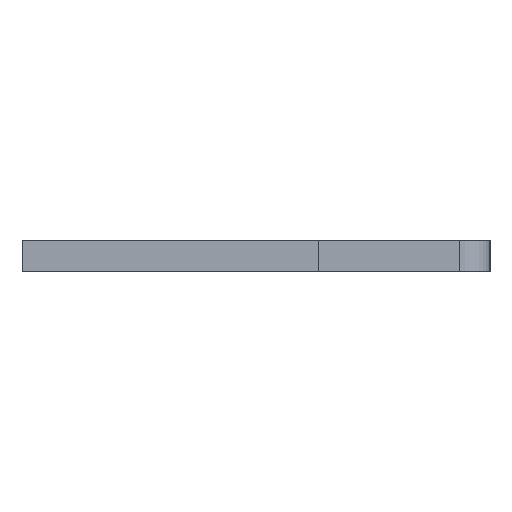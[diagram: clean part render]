
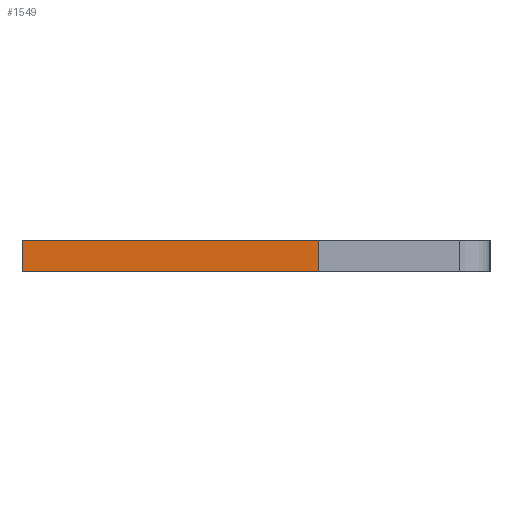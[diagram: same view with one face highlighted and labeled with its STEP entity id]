
A CAD part, left-side view. The second image highlights one B-rep face of the part: STEP entity #1549.
In plain terms, the highlighted face is planar.
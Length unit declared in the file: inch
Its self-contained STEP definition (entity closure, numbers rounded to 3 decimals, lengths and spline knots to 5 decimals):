
#20 = CARTESIAN_POINT ( 'NONE',  ( -0.01, 0.15, -0.04 ) ) ;
#60 = CARTESIAN_POINT ( 'NONE',  ( 0.01, 0.15, -0.04 ) ) ;
#289 = LINE ( 'NONE', #20, #526 ) ;
#394 = LINE ( 'NONE', #60, #2786 ) ;
#432 = CARTESIAN_POINT ( 'NONE',  ( 0.01, -0.04, -0.04 ) ) ;
#434 = VERTEX_POINT ( 'NONE', #1658 ) ;
#450 = DIRECTION ( 'NONE',  ( 1., 0., 0. ) ) ;
#476 = DIRECTION ( 'NONE',  ( 0., 1., 0. ) ) ;
#503 = ORIENTED_EDGE ( 'NONE', *, *, #1906, .T. ) ;
#526 = VECTOR ( 'NONE', #476, 39.37008 ) ;
#716 = ORIENTED_EDGE ( 'NONE', *, *, #2510, .F. ) ;
#841 = VERTEX_POINT ( 'NONE', #861 ) ;
#842 = VECTOR ( 'NONE', #1188, 39.37008 ) ;
#861 = CARTESIAN_POINT ( 'NONE',  ( 0.01, -0.04, -0.04 ) ) ;
#869 = DIRECTION ( 'NONE',  ( -1., 0., 0. ) ) ;
#949 = LINE ( 'NONE', #432, #1327 ) ;
#1083 = PLANE ( 'NONE',  #2396 ) ;
#1135 = CARTESIAN_POINT ( 'NONE',  ( 0.01, 0.15, -0.04 ) ) ;
#1148 = LINE ( 'NONE', #1591, #842 ) ;
#1166 = DIRECTION ( 'NONE',  ( -1., 0., 0. ) ) ;
#1188 = DIRECTION ( 'NONE',  ( 0., 1., 0. ) ) ;
#1327 = VECTOR ( 'NONE', #869, 39.37008 ) ;
#1463 = VERTEX_POINT ( 'NONE', #2209 ) ;
#1549 = ADVANCED_FACE ( 'NONE', ( #2098 ), #1083, .F. ) ;
#1563 = CARTESIAN_POINT ( 'NONE',  ( 0.01, 0.15, -0.04 ) ) ;
#1567 = EDGE_CURVE ( 'NONE', #841, #434, #949, .T. ) ;
#1591 = CARTESIAN_POINT ( 'NONE',  ( 0.01, 0.15, -0.04 ) ) ;
#1658 = CARTESIAN_POINT ( 'NONE',  ( -0.01, -0.04, -0.04 ) ) ;
#1662 = ORIENTED_EDGE ( 'NONE', *, *, #1567, .T. ) ;
#1906 = EDGE_CURVE ( 'NONE', #434, #1463, #289, .T. ) ;
#2018 = EDGE_CURVE ( 'NONE', #2170, #1463, #394, .T. ) ;
#2098 = FACE_OUTER_BOUND ( 'NONE', #2418, .T. ) ;
#2170 = VERTEX_POINT ( 'NONE', #1135 ) ;
#2209 = CARTESIAN_POINT ( 'NONE',  ( -0.01, 0.15, -0.04 ) ) ;
#2288 = ORIENTED_EDGE ( 'NONE', *, *, #2018, .F. ) ;
#2396 = AXIS2_PLACEMENT_3D ( 'NONE', #1563, #2636, #450 ) ;
#2418 = EDGE_LOOP ( 'NONE', ( #503, #2288, #716, #1662 ) ) ;
#2510 = EDGE_CURVE ( 'NONE', #841, #2170, #1148, .T. ) ;
#2636 = DIRECTION ( 'NONE',  ( 0., 0., 1. ) ) ;
#2786 = VECTOR ( 'NONE', #1166, 39.37008 ) ;
